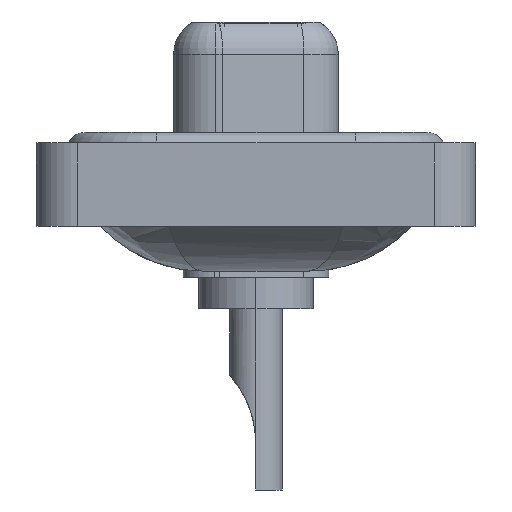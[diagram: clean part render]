
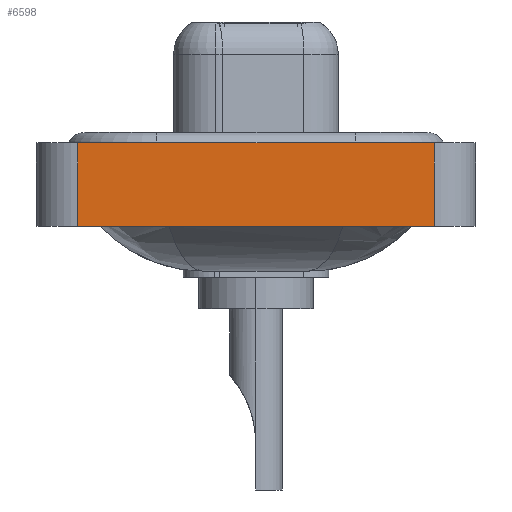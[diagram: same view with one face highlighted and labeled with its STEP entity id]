
A CAD part, left-side view. The second image highlights one B-rep face of the part: STEP entity #6598.
In plain terms, the highlighted planar face has unit normal (-1, 0, 0).
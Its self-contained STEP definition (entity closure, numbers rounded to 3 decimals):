
#905 = ORIENTED_EDGE ( 'NONE', *, *, #16122, .T. ) ;
#1383 = EDGE_CURVE ( 'NONE', #6677, #16466, #11179, .T. ) ;
#2685 = LINE ( 'NONE', #11724, #4292 ) ;
#4184 = CARTESIAN_POINT ( 'NONE',  ( -7.35, 8.55, -3.6 ) ) ;
#4221 = VECTOR ( 'NONE', #11119, 1000. ) ;
#4292 = VECTOR ( 'NONE', #11488, 1000. ) ;
#4722 = EDGE_LOOP ( 'NONE', ( #905, #9351, #9613, #12760 ) ) ;
#5382 = AXIS2_PLACEMENT_3D ( 'NONE', #15961, #12058, #15880 ) ;
#5416 = CARTESIAN_POINT ( 'NONE',  ( -7.35, -8.55, -3.6 ) ) ;
#6161 = CARTESIAN_POINT ( 'NONE',  ( -7.35, -8.55, -3.6 ) ) ;
#6598 = ADVANCED_FACE ( 'NONE', ( #14398 ), #8060, .T. ) ;
#6677 = VERTEX_POINT ( 'NONE', #4184 ) ;
#7099 = EDGE_CURVE ( 'NONE', #12683, #14693, #7176, .T. ) ;
#7176 = LINE ( 'NONE', #12277, #11554 ) ;
#8060 = PLANE ( 'NONE',  #5382 ) ;
#8524 = DIRECTION ( 'NONE',  ( 0., -1., 0. ) ) ;
#8704 = CARTESIAN_POINT ( 'NONE',  ( -7.35, -8.55, -3.6 ) ) ;
#9351 = ORIENTED_EDGE ( 'NONE', *, *, #7099, .F. ) ;
#9613 = ORIENTED_EDGE ( 'NONE', *, *, #13067, .F. ) ;
#11119 = DIRECTION ( 'NONE',  ( 0., 0., 1. ) ) ;
#11179 = LINE ( 'NONE', #6161, #14908 ) ;
#11488 = DIRECTION ( 'NONE',  ( 0., 0., 1. ) ) ;
#11554 = VECTOR ( 'NONE', #8524, 1000. ) ;
#11724 = CARTESIAN_POINT ( 'NONE',  ( -7.35, 8.55, -3.6 ) ) ;
#12058 = DIRECTION ( 'NONE',  ( -1., 0., 0. ) ) ;
#12277 = CARTESIAN_POINT ( 'NONE',  ( -7.35, -8.55, 0.4 ) ) ;
#12408 = CARTESIAN_POINT ( 'NONE',  ( -7.35, -8.55, 0.4 ) ) ;
#12683 = VERTEX_POINT ( 'NONE', #14411 ) ;
#12760 = ORIENTED_EDGE ( 'NONE', *, *, #1383, .T. ) ;
#13067 = EDGE_CURVE ( 'NONE', #6677, #12683, #2685, .T. ) ;
#13871 = LINE ( 'NONE', #8704, #4221 ) ;
#14398 = FACE_OUTER_BOUND ( 'NONE', #4722, .T. ) ;
#14411 = CARTESIAN_POINT ( 'NONE',  ( -7.35, 8.55, 0.4 ) ) ;
#14693 = VERTEX_POINT ( 'NONE', #12408 ) ;
#14908 = VECTOR ( 'NONE', #16341, 1000. ) ;
#15880 = DIRECTION ( 'NONE',  ( 0., 0., 1. ) ) ;
#15961 = CARTESIAN_POINT ( 'NONE',  ( -7.35, -8.55, -3.6 ) ) ;
#16122 = EDGE_CURVE ( 'NONE', #16466, #14693, #13871, .T. ) ;
#16341 = DIRECTION ( 'NONE',  ( 0., -1., 0. ) ) ;
#16466 = VERTEX_POINT ( 'NONE', #5416 ) ;
